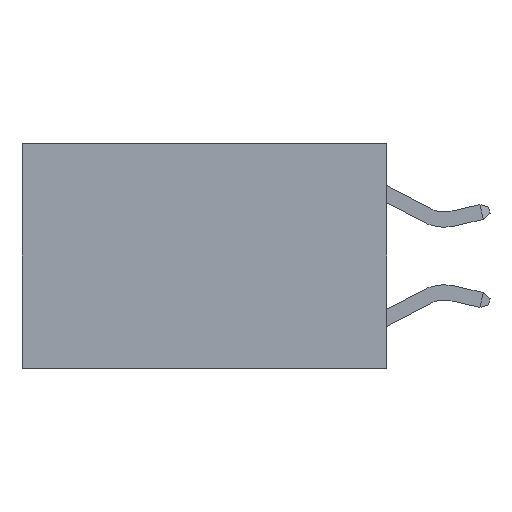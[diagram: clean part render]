
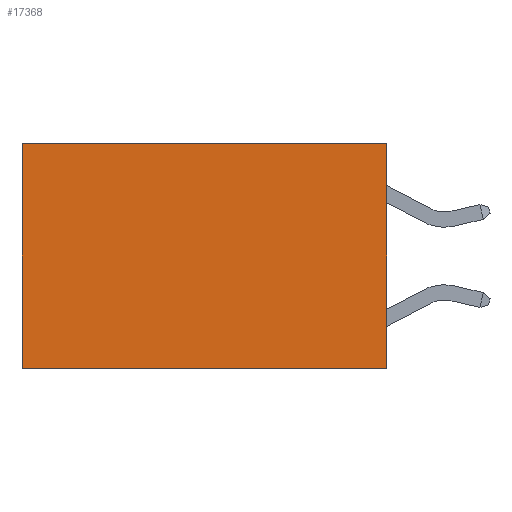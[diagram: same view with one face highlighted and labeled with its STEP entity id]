
A CAD part, left-side view. The second image highlights one B-rep face of the part: STEP entity #17368.
In plain terms, the highlighted planar face has unit normal (-1, 0, 0).
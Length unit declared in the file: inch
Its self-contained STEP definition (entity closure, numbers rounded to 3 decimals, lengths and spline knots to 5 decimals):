
#921 = VECTOR ( 'NONE', #7549, 39.37008 ) ;
#2485 = EDGE_CURVE ( 'NONE', #4128, #15864, #21487, .T. ) ;
#2699 = EDGE_CURVE ( 'NONE', #7053, #6511, #11681, .T. ) ;
#3116 = CARTESIAN_POINT ( 'NONE',  ( 0.2625, 0., -0.37 ) ) ;
#3357 = VECTOR ( 'NONE', #16386, 39.37008 ) ;
#3660 = ORIENTED_EDGE ( 'NONE', *, *, #2485, .F. ) ;
#4128 = VERTEX_POINT ( 'NONE', #16685 ) ;
#4914 = DIRECTION ( 'NONE',  ( 0., 0., -1. ) ) ;
#5705 = LINE ( 'NONE', #14775, #3357 ) ;
#6494 = VECTOR ( 'NONE', #16965, 39.37008 ) ;
#6511 = VERTEX_POINT ( 'NONE', #18477 ) ;
#7053 = VERTEX_POINT ( 'NONE', #14984 ) ;
#7549 = DIRECTION ( 'NONE',  ( 0., 0., -1. ) ) ;
#7793 = EDGE_CURVE ( 'NONE', #15864, #6511, #16082, .T. ) ;
#8127 = EDGE_CURVE ( 'NONE', #4128, #7053, #5705, .T. ) ;
#9105 = AXIS2_PLACEMENT_3D ( 'NONE', #10061, #17084, #4914 ) ;
#9725 = ORIENTED_EDGE ( 'NONE', *, *, #7793, .F. ) ;
#10061 = CARTESIAN_POINT ( 'NONE',  ( 0.2625, 0., 0. ) ) ;
#11570 = FACE_OUTER_BOUND ( 'NONE', #19601, .T. ) ;
#11681 = LINE ( 'NONE', #22284, #6494 ) ;
#14359 = DIRECTION ( 'NONE',  ( 0., 1., 0. ) ) ;
#14590 = ORIENTED_EDGE ( 'NONE', *, *, #8127, .T. ) ;
#14775 = CARTESIAN_POINT ( 'NONE',  ( 0.2625, 0., 0. ) ) ;
#14791 = CARTESIAN_POINT ( 'NONE',  ( 0.2625, 0., 0. ) ) ;
#14984 = CARTESIAN_POINT ( 'NONE',  ( 0.2625, 0.6, 0. ) ) ;
#15864 = VERTEX_POINT ( 'NONE', #3116 ) ;
#16082 = LINE ( 'NONE', #16186, #20232 ) ;
#16186 = CARTESIAN_POINT ( 'NONE',  ( 0.2625, 0., -0.37 ) ) ;
#16386 = DIRECTION ( 'NONE',  ( 0., 1., 0. ) ) ;
#16685 = CARTESIAN_POINT ( 'NONE',  ( 0.2625, 0., 0. ) ) ;
#16965 = DIRECTION ( 'NONE',  ( 0., 0., -1. ) ) ;
#17084 = DIRECTION ( 'NONE',  ( 1., 0., 0. ) ) ;
#17368 = ADVANCED_FACE ( 'NONE', ( #11570 ), #18591, .F. ) ;
#18477 = CARTESIAN_POINT ( 'NONE',  ( 0.2625, 0.6, -0.37 ) ) ;
#18591 = PLANE ( 'NONE',  #9105 ) ;
#19601 = EDGE_LOOP ( 'NONE', ( #21164, #9725, #3660, #14590 ) ) ;
#20232 = VECTOR ( 'NONE', #14359, 39.37008 ) ;
#21164 = ORIENTED_EDGE ( 'NONE', *, *, #2699, .T. ) ;
#21487 = LINE ( 'NONE', #14791, #921 ) ;
#22284 = CARTESIAN_POINT ( 'NONE',  ( 0.2625, 0.6, 0. ) ) ;
